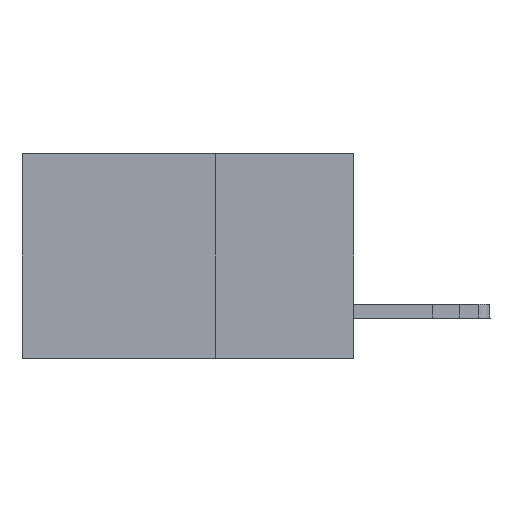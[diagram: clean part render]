
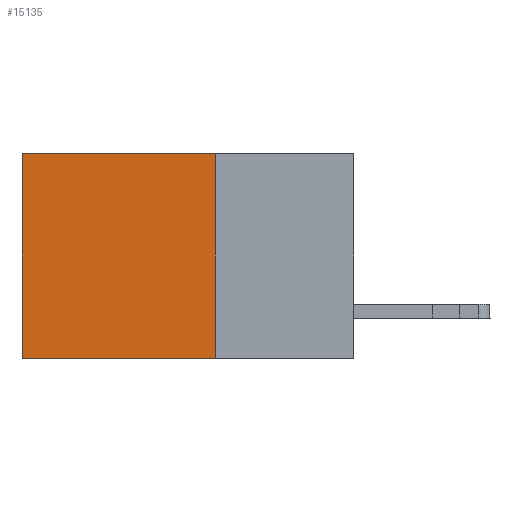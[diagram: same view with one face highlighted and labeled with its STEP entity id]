
A CAD part, left-side view. The second image highlights one B-rep face of the part: STEP entity #15135.
In plain terms, the highlighted planar face has unit normal (-1, 0, 0).
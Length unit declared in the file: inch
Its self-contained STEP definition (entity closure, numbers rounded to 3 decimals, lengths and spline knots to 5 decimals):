
#1243 = CARTESIAN_POINT ( 'NONE',  ( 0.2875, 0.25, 0. ) ) ;
#1286 = VECTOR ( 'NONE', #9171, 39.37008 ) ;
#1318 = LINE ( 'NONE', #15797, #14245 ) ;
#1693 = LINE ( 'NONE', #10457, #1286 ) ;
#1929 = CARTESIAN_POINT ( 'NONE',  ( 0.2875, 0.6, 0. ) ) ;
#1964 = EDGE_CURVE ( 'NONE', #2179, #5524, #12010, .T. ) ;
#2179 = VERTEX_POINT ( 'NONE', #10382 ) ;
#2536 = VERTEX_POINT ( 'NONE', #3315 ) ;
#3315 = CARTESIAN_POINT ( 'NONE',  ( 0.2875, 0.6, -0.37 ) ) ;
#3359 = DIRECTION ( 'NONE',  ( 0., 1., 0. ) ) ;
#4127 = DIRECTION ( 'NONE',  ( 1., 0., 0. ) ) ;
#4301 = DIRECTION ( 'NONE',  ( 0., 1., 0. ) ) ;
#4325 = DIRECTION ( 'NONE',  ( 0., 0., -1. ) ) ;
#4950 = VECTOR ( 'NONE', #4301, 39.37008 ) ;
#5524 = VERTEX_POINT ( 'NONE', #1929 ) ;
#6869 = CARTESIAN_POINT ( 'NONE',  ( 0.2875, 0.25, 0. ) ) ;
#7158 = EDGE_CURVE ( 'NONE', #13528, #2536, #1318, .T. ) ;
#7505 = AXIS2_PLACEMENT_3D ( 'NONE', #10423, #4127, #12856 ) ;
#7977 = ORIENTED_EDGE ( 'NONE', *, *, #8707, .T. ) ;
#8167 = ORIENTED_EDGE ( 'NONE', *, *, #7158, .F. ) ;
#8196 = ORIENTED_EDGE ( 'NONE', *, *, #8832, .F. ) ;
#8214 = ORIENTED_EDGE ( 'NONE', *, *, #1964, .T. ) ;
#8707 = EDGE_CURVE ( 'NONE', #5524, #2536, #1693, .T. ) ;
#8832 = EDGE_CURVE ( 'NONE', #2179, #13528, #15900, .T. ) ;
#9171 = DIRECTION ( 'NONE',  ( 0., 0., -1. ) ) ;
#9425 = VECTOR ( 'NONE', #4325, 39.37008 ) ;
#10382 = CARTESIAN_POINT ( 'NONE',  ( 0.2875, 0.25, 0. ) ) ;
#10423 = CARTESIAN_POINT ( 'NONE',  ( 0.2875, 0.25, 0. ) ) ;
#10457 = CARTESIAN_POINT ( 'NONE',  ( 0.2875, 0.6, 0. ) ) ;
#12010 = LINE ( 'NONE', #1243, #4950 ) ;
#12856 = DIRECTION ( 'NONE',  ( 0., 0., -1. ) ) ;
#13528 = VERTEX_POINT ( 'NONE', #14380 ) ;
#14031 = PLANE ( 'NONE',  #7505 ) ;
#14132 = EDGE_LOOP ( 'NONE', ( #7977, #8167, #8196, #8214 ) ) ;
#14245 = VECTOR ( 'NONE', #3359, 39.37008 ) ;
#14380 = CARTESIAN_POINT ( 'NONE',  ( 0.2875, 0.25, -0.37 ) ) ;
#14513 = FACE_OUTER_BOUND ( 'NONE', #14132, .T. ) ;
#15135 = ADVANCED_FACE ( 'NONE', ( #14513 ), #14031, .F. ) ;
#15797 = CARTESIAN_POINT ( 'NONE',  ( 0.2875, 0.25, -0.37 ) ) ;
#15900 = LINE ( 'NONE', #6869, #9425 ) ;
